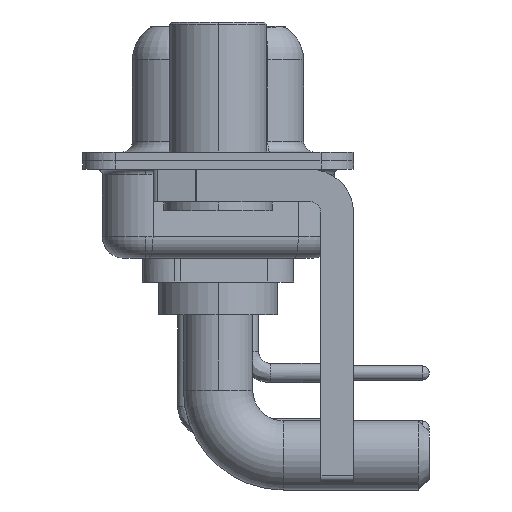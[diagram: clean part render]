
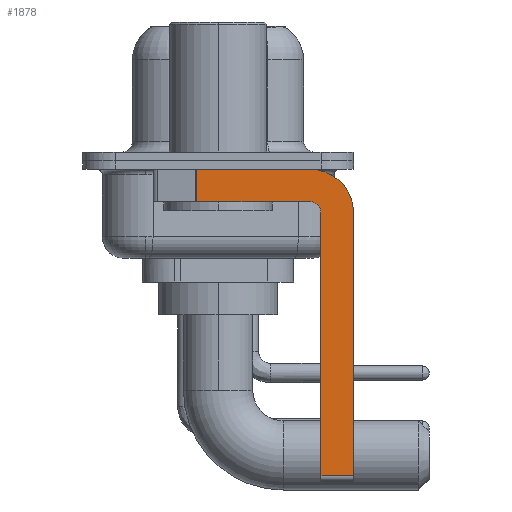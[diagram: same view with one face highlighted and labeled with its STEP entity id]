
A CAD part, left-side view. The second image highlights one B-rep face of the part: STEP entity #1878.
In plain terms, the highlighted planar face has unit normal (-1, 0, 0).
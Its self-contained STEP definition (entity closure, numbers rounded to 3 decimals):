
#412 = VERTEX_POINT ( 'NONE', #18850 ) ;
#818 = VECTOR ( 'NONE', #2700, 1000. ) ;
#865 = CARTESIAN_POINT ( 'NONE',  ( -2.9, -4.25, -2.4 ) ) ;
#1782 = VERTEX_POINT ( 'NONE', #12013 ) ;
#1878 = ADVANCED_FACE ( 'NONE', ( #9138 ), #20125, .F. ) ;
#1995 = DIRECTION ( 'NONE',  ( 0., -1., 0. ) ) ;
#2185 = DIRECTION ( 'NONE',  ( 0., -1., 0. ) ) ;
#2369 = DIRECTION ( 'NONE',  ( -1., 0., 0. ) ) ;
#2420 = ORIENTED_EDGE ( 'NONE', *, *, #14822, .F. ) ;
#2700 = DIRECTION ( 'NONE',  ( 0., 0., -1. ) ) ;
#3214 = VECTOR ( 'NONE', #1995, 1000. ) ;
#3678 = CARTESIAN_POINT ( 'NONE',  ( -2.9, -4.75, -14.55 ) ) ;
#4088 = ORIENTED_EDGE ( 'NONE', *, *, #7953, .F. ) ;
#4302 = DIRECTION ( 'NONE',  ( 0., 0., 1. ) ) ;
#4494 = CARTESIAN_POINT ( 'NONE',  ( -2.9, -4.75, -14.8 ) ) ;
#4549 = DIRECTION ( 'NONE',  ( 1., 0., 0. ) ) ;
#4620 = AXIS2_PLACEMENT_3D ( 'NONE', #18122, #2369, #4302 ) ;
#4927 = CARTESIAN_POINT ( 'NONE',  ( -2.9, -6.25, -14.55 ) ) ;
#5288 = ORIENTED_EDGE ( 'NONE', *, *, #17778, .F. ) ;
#6204 = EDGE_CURVE ( 'NONE', #1782, #21311, #18939, .T. ) ;
#6392 = VERTEX_POINT ( 'NONE', #8657 ) ;
#7262 = DIRECTION ( 'NONE',  ( 0., 1., 0. ) ) ;
#7394 = CARTESIAN_POINT ( 'NONE',  ( -2.9, -6.25, -2.4 ) ) ;
#7832 = CARTESIAN_POINT ( 'NONE',  ( -2.9, -4.25, -2.4 ) ) ;
#7953 = EDGE_CURVE ( 'NONE', #19280, #412, #10744, .T. ) ;
#7985 = LINE ( 'NONE', #8102, #818 ) ;
#8093 = VECTOR ( 'NONE', #2185, 1000. ) ;
#8102 = CARTESIAN_POINT ( 'NONE',  ( -2.9, 0.978, -1.9 ) ) ;
#8178 = LINE ( 'NONE', #4494, #16542 ) ;
#8657 = CARTESIAN_POINT ( 'NONE',  ( -2.9, -6.25, -2.4 ) ) ;
#8725 = VECTOR ( 'NONE', #7262, 1000. ) ;
#8813 = AXIS2_PLACEMENT_3D ( 'NONE', #865, #4549, #16754 ) ;
#9138 = FACE_OUTER_BOUND ( 'NONE', #16410, .T. ) ;
#9667 = VECTOR ( 'NONE', #15914, 1000. ) ;
#9672 = DIRECTION ( 'NONE',  ( 1., 0., 0. ) ) ;
#10241 = EDGE_CURVE ( 'NONE', #18284, #1782, #8178, .T. ) ;
#10744 = LINE ( 'NONE', #21312, #3214 ) ;
#10893 = AXIS2_PLACEMENT_3D ( 'NONE', #7832, #9672, #11286 ) ;
#11082 = LINE ( 'NONE', #7394, #9667 ) ;
#11265 = LINE ( 'NONE', #17940, #8093 ) ;
#11286 = DIRECTION ( 'NONE',  ( 0., 0., -1. ) ) ;
#11419 = CARTESIAN_POINT ( 'NONE',  ( -2.9, -4.25, -1.9 ) ) ;
#11626 = DIRECTION ( 'NONE',  ( 0., 0., 1. ) ) ;
#12013 = CARTESIAN_POINT ( 'NONE',  ( -2.9, -4.75, -2.4 ) ) ;
#12278 = EDGE_CURVE ( 'NONE', #18284, #18044, #11265, .T. ) ;
#14577 = EDGE_CURVE ( 'NONE', #19280, #19175, #7985, .T. ) ;
#14822 = EDGE_CURVE ( 'NONE', #6392, #18044, #11082, .T. ) ;
#15085 = ORIENTED_EDGE ( 'NONE', *, *, #12278, .T. ) ;
#15262 = ORIENTED_EDGE ( 'NONE', *, *, #14577, .T. ) ;
#15583 = ORIENTED_EDGE ( 'NONE', *, *, #20176, .F. ) ;
#15914 = DIRECTION ( 'NONE',  ( 0., 0., -1. ) ) ;
#16410 = EDGE_LOOP ( 'NONE', ( #4088, #15262, #5288, #21318, #21431, #15085, #2420, #15583 ) ) ;
#16542 = VECTOR ( 'NONE', #11626, 1000. ) ;
#16754 = DIRECTION ( 'NONE',  ( 0., 0., -1. ) ) ;
#16804 = CARTESIAN_POINT ( 'NONE',  ( -2.9, 0.978, -0.4 ) ) ;
#17262 = CIRCLE ( 'NONE', #8813, 2. ) ;
#17742 = LINE ( 'NONE', #21401, #8725 ) ;
#17778 = EDGE_CURVE ( 'NONE', #21311, #19175, #17742, .T. ) ;
#17940 = CARTESIAN_POINT ( 'NONE',  ( -2.9, -4.25, -14.55 ) ) ;
#18044 = VERTEX_POINT ( 'NONE', #4927 ) ;
#18122 = CARTESIAN_POINT ( 'NONE',  ( -2.9, -4.25, -2.4 ) ) ;
#18284 = VERTEX_POINT ( 'NONE', #3678 ) ;
#18850 = CARTESIAN_POINT ( 'NONE',  ( -2.9, -4.25, -0.4 ) ) ;
#18939 = CIRCLE ( 'NONE', #4620, 0.5 ) ;
#19175 = VERTEX_POINT ( 'NONE', #21621 ) ;
#19280 = VERTEX_POINT ( 'NONE', #16804 ) ;
#20125 = PLANE ( 'NONE',  #10893 ) ;
#20176 = EDGE_CURVE ( 'NONE', #412, #6392, #17262, .T. ) ;
#21311 = VERTEX_POINT ( 'NONE', #11419 ) ;
#21312 = CARTESIAN_POINT ( 'NONE',  ( -2.9, 3., -0.4 ) ) ;
#21318 = ORIENTED_EDGE ( 'NONE', *, *, #6204, .F. ) ;
#21401 = CARTESIAN_POINT ( 'NONE',  ( -2.9, -4.25, -1.9 ) ) ;
#21431 = ORIENTED_EDGE ( 'NONE', *, *, #10241, .F. ) ;
#21621 = CARTESIAN_POINT ( 'NONE',  ( -2.9, 0.978, -1.9 ) ) ;
